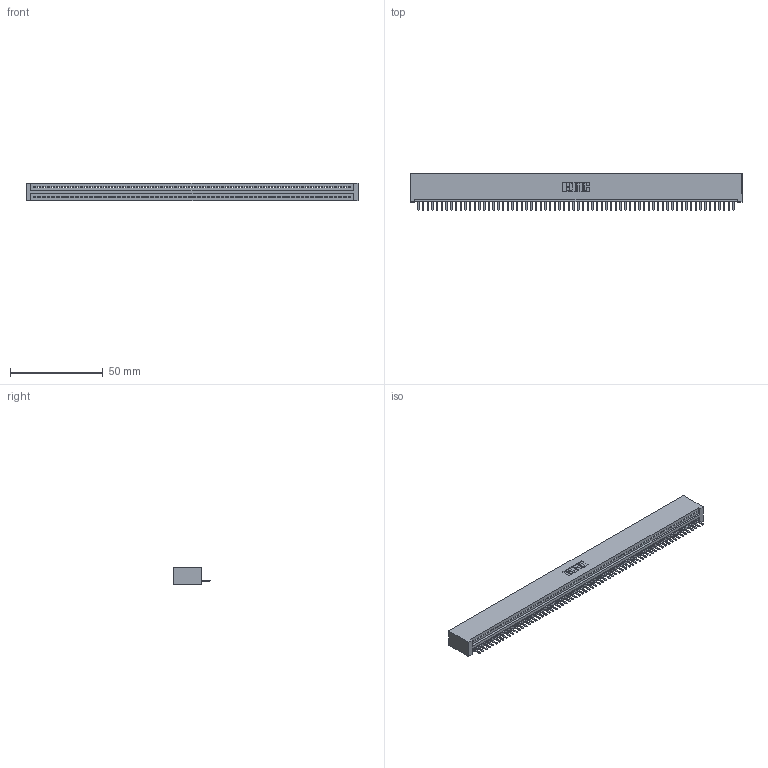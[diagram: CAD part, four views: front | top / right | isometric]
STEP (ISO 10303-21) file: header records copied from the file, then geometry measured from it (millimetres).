
FILE_DESCRIPTION (( 'STEP AP203' ), '1' );
FILE_NAME ('345-068-520-101.STEP', '2018-09-29T06:38:59', ( '' ), ( '' ), 'SwSTEP 2.0', 'SolidWorks 2016', '' );
FILE_SCHEMA (( 'CONFIG_CONTROL_DESIGN' ));
Length unit declared in the file: inch
Products named in the file (3): 345-292-001_345-293-120; 345-068-520-101; 345 Part_No Mounting Lugs
Assembly tree (69 placements, depth 2):
  345-068-520-101
    345 Part_No Mounting Lugs
    345-292-001_345-293-120  x68
Bounding box: 179.32 x 19.68 x 9.4 mm (x, y, z)
Volume: 17634.1 mm3; surface area: 23337.7 mm2
Topology: 69 solids, 69 shells, 4334 faces, 12829 edges, 8370 vertices
Faces by surface type: plane 2932, cylinder 1402
Entity records: 47515 total; most frequent: CARTESIAN_POINT 8248, ORIENTED_EDGE 8238, DIRECTION 7147, EDGE_CURVE 4119, VECTOR 3719, LINE 3719, VERTEX_POINT 2742, AXIS2_PLACEMENT_3D 1714
